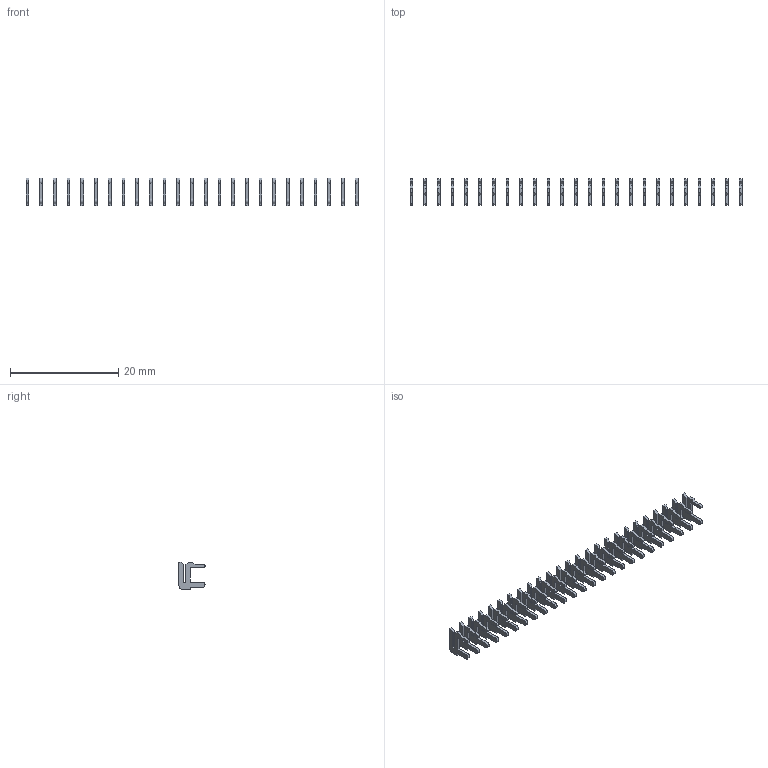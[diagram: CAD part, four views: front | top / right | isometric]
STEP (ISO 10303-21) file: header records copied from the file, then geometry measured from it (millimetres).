
FILE_DESCRIPTION (( 'STEP AP203' ), '1' );
FILE_NAME ('105-025-208-100.STEP', '2020-04-07T23:12:40', ( '' ), ( '' ), 'SwSTEP 2.0', 'SolidWorks 2016', '' );
FILE_SCHEMA (( 'CONFIG_CONTROL_DESIGN' ));
Length unit declared in the file: inch
Products named in the file (2): 100-290-001_100-290-208; 105-025-208-100
Assembly tree (25 placements, depth 2):
  105-025-208-100
    100-290-001_100-290-208  x25
Bounding box: 61.47 x 4.83 x 5.17 mm (x, y, z)
Volume: 172 mm3; surface area: 1062.4 mm2
Topology: 25 solids, 25 shells, 625 faces, 1725 edges, 1150 vertices
Faces by surface type: plane 550, cylinder 75
Entity records: 1757 total; most frequent: DIRECTION 181, CARTESIAN_POINT 168, ORIENTED_EDGE 138, EDGE_CURVE 69, VECTOR 63, LINE 63, DATE_AND_TIME 60, CALENDAR_DATE 60
